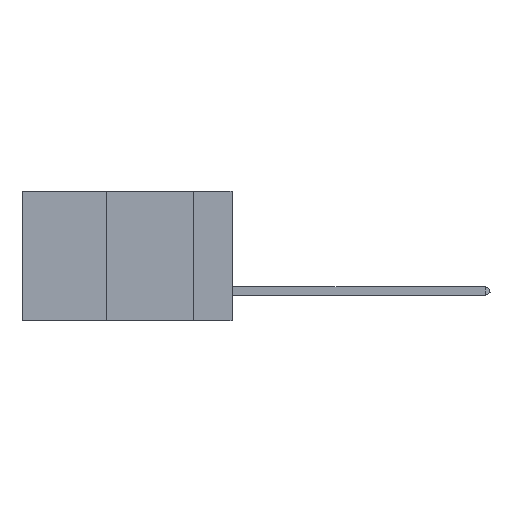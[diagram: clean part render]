
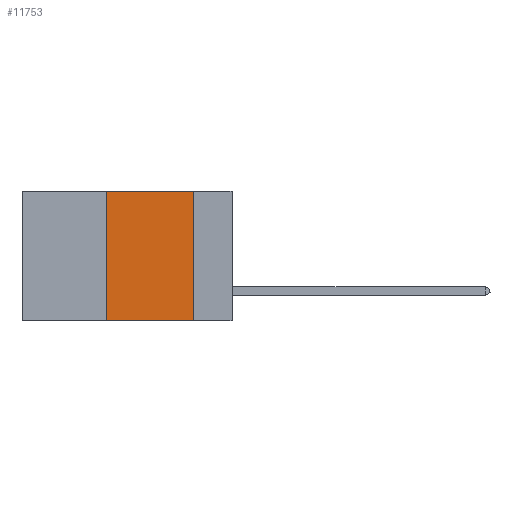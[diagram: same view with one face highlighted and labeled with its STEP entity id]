
A CAD part, left-side view. The second image highlights one B-rep face of the part: STEP entity #11753.
In plain terms, the highlighted planar face has unit normal (-1, 0, 0).
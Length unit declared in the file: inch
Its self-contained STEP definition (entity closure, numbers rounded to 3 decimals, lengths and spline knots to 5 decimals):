
#263 = VERTEX_POINT ( 'NONE', #4590 ) ;
#651 = EDGE_CURVE ( 'NONE', #263, #7026, #3117, .T. ) ;
#872 = CARTESIAN_POINT ( 'NONE',  ( 0., 0.6, 0. ) ) ;
#1163 = ORIENTED_EDGE ( 'NONE', *, *, #10393, .F. ) ;
#1244 = ORIENTED_EDGE ( 'NONE', *, *, #651, .F. ) ;
#1705 = LINE ( 'NONE', #6122, #11077 ) ;
#2002 = AXIS2_PLACEMENT_3D ( 'NONE', #3103, #6609, #8534 ) ;
#2282 = VERTEX_POINT ( 'NONE', #8448 ) ;
#3103 = CARTESIAN_POINT ( 'NONE',  ( 0., 0.6, 0. ) ) ;
#3117 = LINE ( 'NONE', #3959, #8929 ) ;
#3959 = CARTESIAN_POINT ( 'NONE',  ( 0., 0.36, 0. ) ) ;
#4408 = CARTESIAN_POINT ( 'NONE',  ( 0., 0.11, 0. ) ) ;
#4442 = DIRECTION ( 'NONE',  ( 0., -1., 0. ) ) ;
#4590 = CARTESIAN_POINT ( 'NONE',  ( 0., 0.36, -0.37 ) ) ;
#4745 = ORIENTED_EDGE ( 'NONE', *, *, #10458, .F. ) ;
#5567 = DIRECTION ( 'NONE',  ( 0., 0., 1. ) ) ;
#5984 = VERTEX_POINT ( 'NONE', #8437 ) ;
#5999 = EDGE_LOOP ( 'NONE', ( #4745, #1163, #1244, #7094 ) ) ;
#6108 = FACE_OUTER_BOUND ( 'NONE', #5999, .T. ) ;
#6122 = CARTESIAN_POINT ( 'NONE',  ( 0., 0.6, -0.37 ) ) ;
#6609 = DIRECTION ( 'NONE',  ( 1., 0., 0. ) ) ;
#6866 = VECTOR ( 'NONE', #9801, 39.37008 ) ;
#7026 = VERTEX_POINT ( 'NONE', #11375 ) ;
#7094 = ORIENTED_EDGE ( 'NONE', *, *, #8245, .T. ) ;
#8245 = EDGE_CURVE ( 'NONE', #263, #5984, #1705, .T. ) ;
#8437 = CARTESIAN_POINT ( 'NONE',  ( 0., 0.11, -0.37 ) ) ;
#8448 = CARTESIAN_POINT ( 'NONE',  ( 0., 0.11, 0. ) ) ;
#8534 = DIRECTION ( 'NONE',  ( 0., 0., -1. ) ) ;
#8721 = VECTOR ( 'NONE', #10687, 39.37008 ) ;
#8929 = VECTOR ( 'NONE', #5567, 39.37008 ) ;
#9423 = LINE ( 'NONE', #4408, #8721 ) ;
#9801 = DIRECTION ( 'NONE',  ( 0., -1., 0. ) ) ;
#10361 = PLANE ( 'NONE',  #2002 ) ;
#10393 = EDGE_CURVE ( 'NONE', #7026, #2282, #11431, .T. ) ;
#10458 = EDGE_CURVE ( 'NONE', #2282, #5984, #9423, .T. ) ;
#10687 = DIRECTION ( 'NONE',  ( 0., 0., -1. ) ) ;
#11077 = VECTOR ( 'NONE', #4442, 39.37008 ) ;
#11375 = CARTESIAN_POINT ( 'NONE',  ( 0., 0.36, 0. ) ) ;
#11431 = LINE ( 'NONE', #872, #6866 ) ;
#11753 = ADVANCED_FACE ( 'NONE', ( #6108 ), #10361, .F. ) ;
